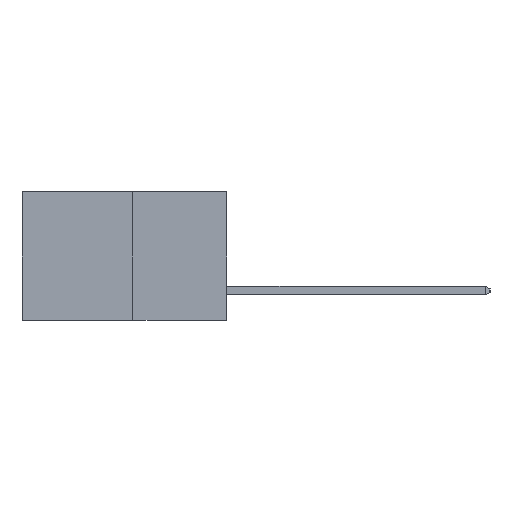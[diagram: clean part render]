
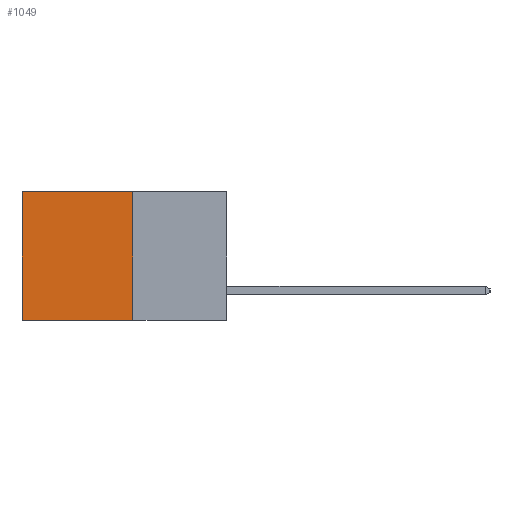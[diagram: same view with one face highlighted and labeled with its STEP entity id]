
A CAD part, left-side view. The second image highlights one B-rep face of the part: STEP entity #1049.
In plain terms, the highlighted planar face has unit normal (-1, 0, 0).
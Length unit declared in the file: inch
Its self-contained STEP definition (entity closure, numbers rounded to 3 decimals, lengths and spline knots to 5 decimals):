
#819 = DIRECTION ( 'NONE',  ( 0., 0., -1. ) ) ;
#1049 = ADVANCED_FACE ( 'NONE', ( #11254 ), #9927, .F. ) ;
#1150 = EDGE_CURVE ( 'NONE', #6986, #13179, #2149, .T. ) ;
#1506 = VECTOR ( 'NONE', #10082, 39.37008 ) ;
#2149 = LINE ( 'NONE', #5552, #13406 ) ;
#2195 = ORIENTED_EDGE ( 'NONE', *, *, #14279, .T. ) ;
#3825 = AXIS2_PLACEMENT_3D ( 'NONE', #6898, #9991, #819 ) ;
#4558 = CARTESIAN_POINT ( 'NONE',  ( 0.277, 0.27, 0. ) ) ;
#4786 = CARTESIAN_POINT ( 'NONE',  ( 0.277, 0.59, 0. ) ) ;
#4950 = CARTESIAN_POINT ( 'NONE',  ( 0.277, 0.27, -0.37 ) ) ;
#5096 = LINE ( 'NONE', #19217, #1506 ) ;
#5153 = LINE ( 'NONE', #14504, #12836 ) ;
#5552 = CARTESIAN_POINT ( 'NONE',  ( 0.277, 0.27, -0.37 ) ) ;
#6112 = DIRECTION ( 'NONE',  ( 0., 1., 0. ) ) ;
#6898 = CARTESIAN_POINT ( 'NONE',  ( 0.277, 0.27, -0.37 ) ) ;
#6986 = VERTEX_POINT ( 'NONE', #4950 ) ;
#8528 = VECTOR ( 'NONE', #6112, 39.37008 ) ;
#9146 = CARTESIAN_POINT ( 'NONE',  ( 0.277, 0.27, 0. ) ) ;
#9648 = EDGE_CURVE ( 'NONE', #11286, #13179, #5153, .T. ) ;
#9927 = PLANE ( 'NONE',  #3825 ) ;
#9991 = DIRECTION ( 'NONE',  ( 1., 0., 0. ) ) ;
#10082 = DIRECTION ( 'NONE',  ( 0., 0., -1. ) ) ;
#10186 = DIRECTION ( 'NONE',  ( 0., 1., 0. ) ) ;
#11254 = FACE_OUTER_BOUND ( 'NONE', #12902, .T. ) ;
#11286 = VERTEX_POINT ( 'NONE', #4786 ) ;
#11579 = EDGE_CURVE ( 'NONE', #13200, #6986, #5096, .T. ) ;
#12766 = ORIENTED_EDGE ( 'NONE', *, *, #1150, .F. ) ;
#12836 = VECTOR ( 'NONE', #12991, 39.37008 ) ;
#12902 = EDGE_LOOP ( 'NONE', ( #17611, #12766, #17949, #2195 ) ) ;
#12991 = DIRECTION ( 'NONE',  ( 0., 0., -1. ) ) ;
#13179 = VERTEX_POINT ( 'NONE', #16700 ) ;
#13200 = VERTEX_POINT ( 'NONE', #9146 ) ;
#13406 = VECTOR ( 'NONE', #10186, 39.37008 ) ;
#14279 = EDGE_CURVE ( 'NONE', #13200, #11286, #16669, .T. ) ;
#14504 = CARTESIAN_POINT ( 'NONE',  ( 0.277, 0.59, -0.37 ) ) ;
#16669 = LINE ( 'NONE', #4558, #8528 ) ;
#16700 = CARTESIAN_POINT ( 'NONE',  ( 0.277, 0.59, -0.37 ) ) ;
#17611 = ORIENTED_EDGE ( 'NONE', *, *, #9648, .T. ) ;
#17949 = ORIENTED_EDGE ( 'NONE', *, *, #11579, .F. ) ;
#19217 = CARTESIAN_POINT ( 'NONE',  ( 0.277, 0.27, -0.37 ) ) ;
